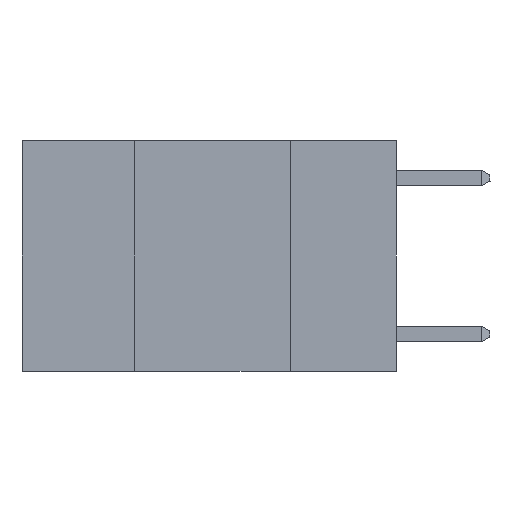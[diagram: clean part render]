
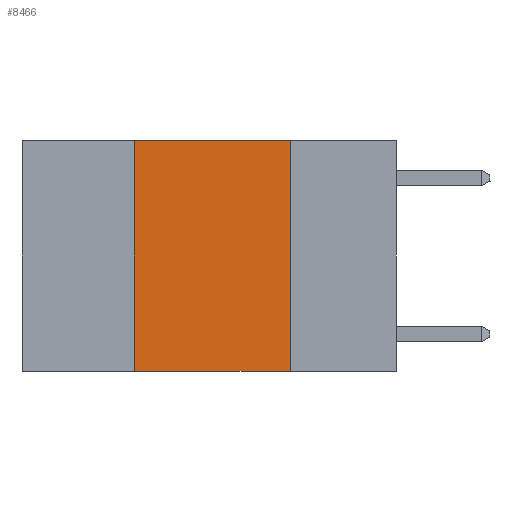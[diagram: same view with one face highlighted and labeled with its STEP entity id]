
A CAD part, left-side view. The second image highlights one B-rep face of the part: STEP entity #8466.
In plain terms, the highlighted planar face has unit normal (-1, 0, 0).
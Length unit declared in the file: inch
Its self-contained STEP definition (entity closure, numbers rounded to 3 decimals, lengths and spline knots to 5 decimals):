
#1645 = EDGE_CURVE ( 'NONE', #16905, #8848, #12722, .T. ) ;
#2835 = DIRECTION ( 'NONE',  ( 0., -1., 0. ) ) ;
#2868 = DIRECTION ( 'NONE',  ( 0., 0., 1. ) ) ;
#2975 = CARTESIAN_POINT ( 'NONE',  ( 0., 0.17, -0.37 ) ) ;
#4345 = CARTESIAN_POINT ( 'NONE',  ( 0., 0.17, 0. ) ) ;
#4393 = VERTEX_POINT ( 'NONE', #4345 ) ;
#4848 = AXIS2_PLACEMENT_3D ( 'NONE', #22677, #18915, #7502 ) ;
#5545 = PLANE ( 'NONE',  #4848 ) ;
#5955 = ORIENTED_EDGE ( 'NONE', *, *, #1645, .T. ) ;
#6406 = CARTESIAN_POINT ( 'NONE',  ( 0., 0.42, 0. ) ) ;
#7502 = DIRECTION ( 'NONE',  ( 0., 0., -1. ) ) ;
#7660 = VECTOR ( 'NONE', #20585, 39.37008 ) ;
#8466 = ADVANCED_FACE ( 'NONE', ( #18992 ), #5545, .F. ) ;
#8776 = CARTESIAN_POINT ( 'NONE',  ( 0., 0.6, -0.37 ) ) ;
#8848 = VERTEX_POINT ( 'NONE', #2975 ) ;
#9506 = LINE ( 'NONE', #12436, #13991 ) ;
#12213 = ORIENTED_EDGE ( 'NONE', *, *, #14372, .F. ) ;
#12436 = CARTESIAN_POINT ( 'NONE',  ( 0., 0.6, 0. ) ) ;
#12722 = LINE ( 'NONE', #8776, #7660 ) ;
#13991 = VECTOR ( 'NONE', #2835, 39.37008 ) ;
#14372 = EDGE_CURVE ( 'NONE', #4393, #8848, #21471, .T. ) ;
#14644 = VECTOR ( 'NONE', #2868, 39.37008 ) ;
#15843 = VECTOR ( 'NONE', #24559, 39.37008 ) ;
#16905 = VERTEX_POINT ( 'NONE', #17152 ) ;
#17152 = CARTESIAN_POINT ( 'NONE',  ( 0., 0.42, -0.37 ) ) ;
#17945 = ORIENTED_EDGE ( 'NONE', *, *, #21256, .F. ) ;
#18305 = VERTEX_POINT ( 'NONE', #6406 ) ;
#18450 = EDGE_LOOP ( 'NONE', ( #12213, #17945, #24247, #5955 ) ) ;
#18915 = DIRECTION ( 'NONE',  ( 1., 0., 0. ) ) ;
#18992 = FACE_OUTER_BOUND ( 'NONE', #18450, .T. ) ;
#19640 = EDGE_CURVE ( 'NONE', #16905, #18305, #24793, .T. ) ;
#20127 = CARTESIAN_POINT ( 'NONE',  ( 0., 0.42, 0. ) ) ;
#20585 = DIRECTION ( 'NONE',  ( 0., -1., 0. ) ) ;
#21256 = EDGE_CURVE ( 'NONE', #18305, #4393, #9506, .T. ) ;
#21471 = LINE ( 'NONE', #22595, #15843 ) ;
#22595 = CARTESIAN_POINT ( 'NONE',  ( 0., 0.17, 0. ) ) ;
#22677 = CARTESIAN_POINT ( 'NONE',  ( 0., 0.6, 0. ) ) ;
#24247 = ORIENTED_EDGE ( 'NONE', *, *, #19640, .F. ) ;
#24559 = DIRECTION ( 'NONE',  ( 0., 0., -1. ) ) ;
#24793 = LINE ( 'NONE', #20127, #14644 ) ;
